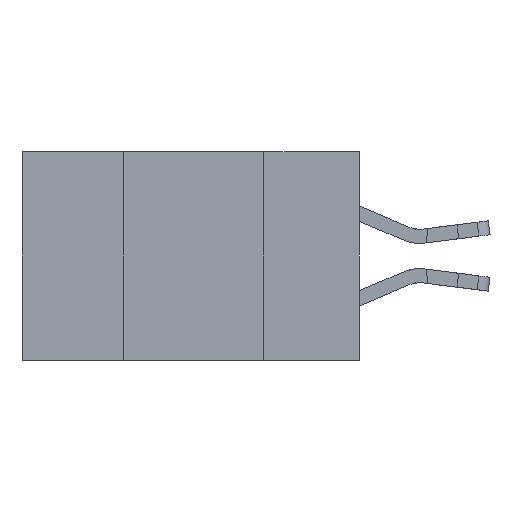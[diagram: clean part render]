
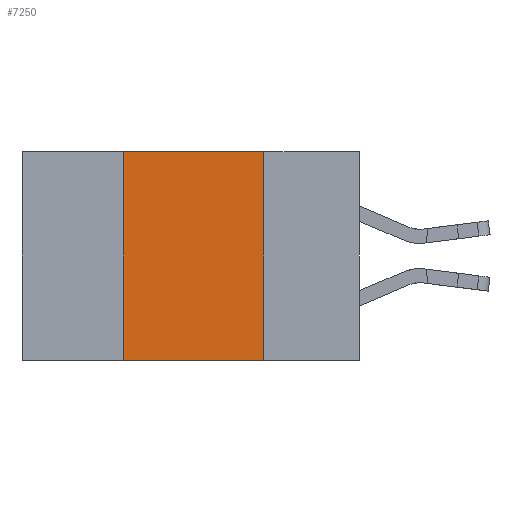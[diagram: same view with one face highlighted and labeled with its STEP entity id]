
A CAD part, left-side view. The second image highlights one B-rep face of the part: STEP entity #7250.
In plain terms, the highlighted planar face has unit normal (-1, 0, 0).
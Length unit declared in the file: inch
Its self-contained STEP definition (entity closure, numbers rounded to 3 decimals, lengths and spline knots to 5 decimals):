
#182 = LINE ( 'NONE', #4715, #15017 ) ;
#208 = VERTEX_POINT ( 'NONE', #18046 ) ;
#451 = EDGE_CURVE ( 'NONE', #5665, #13967, #7849, .T. ) ;
#757 = CARTESIAN_POINT ( 'NONE',  ( 0., 0.6, 0. ) ) ;
#1603 = DIRECTION ( 'NONE',  ( 0., 0., -1. ) ) ;
#2274 = CARTESIAN_POINT ( 'NONE',  ( 0., 0.42, 0. ) ) ;
#3201 = LINE ( 'NONE', #2274, #12126 ) ;
#3503 = VECTOR ( 'NONE', #9624, 39.37008 ) ;
#4179 = ORIENTED_EDGE ( 'NONE', *, *, #10202, .T. ) ;
#4546 = CARTESIAN_POINT ( 'NONE',  ( 0., 0.17, 0. ) ) ;
#4715 = CARTESIAN_POINT ( 'NONE',  ( 0., 0.17, 0. ) ) ;
#5426 = EDGE_LOOP ( 'NONE', ( #12099, #19490, #9662, #4179 ) ) ;
#5665 = VERTEX_POINT ( 'NONE', #16697 ) ;
#6869 = VECTOR ( 'NONE', #13928, 39.37008 ) ;
#7250 = ADVANCED_FACE ( 'NONE', ( #10138 ), #18118, .F. ) ;
#7813 = EDGE_CURVE ( 'NONE', #13967, #208, #182, .T. ) ;
#7849 = LINE ( 'NONE', #12889, #6869 ) ;
#8028 = CARTESIAN_POINT ( 'NONE',  ( 0., 0.6, -0.37 ) ) ;
#8207 = LINE ( 'NONE', #8028, #3503 ) ;
#8714 = DIRECTION ( 'NONE',  ( 1., 0., 0. ) ) ;
#9403 = AXIS2_PLACEMENT_3D ( 'NONE', #757, #8714, #19716 ) ;
#9497 = CARTESIAN_POINT ( 'NONE',  ( 0., 0.42, -0.37 ) ) ;
#9624 = DIRECTION ( 'NONE',  ( 0., -1., 0. ) ) ;
#9662 = ORIENTED_EDGE ( 'NONE', *, *, #13712, .F. ) ;
#10138 = FACE_OUTER_BOUND ( 'NONE', #5426, .T. ) ;
#10202 = EDGE_CURVE ( 'NONE', #17952, #208, #8207, .T. ) ;
#11749 = DIRECTION ( 'NONE',  ( 0., 0., 1. ) ) ;
#12099 = ORIENTED_EDGE ( 'NONE', *, *, #7813, .F. ) ;
#12126 = VECTOR ( 'NONE', #11749, 39.37008 ) ;
#12889 = CARTESIAN_POINT ( 'NONE',  ( 0., 0.6, 0. ) ) ;
#13712 = EDGE_CURVE ( 'NONE', #17952, #5665, #3201, .T. ) ;
#13928 = DIRECTION ( 'NONE',  ( 0., -1., 0. ) ) ;
#13967 = VERTEX_POINT ( 'NONE', #4546 ) ;
#15017 = VECTOR ( 'NONE', #1603, 39.37008 ) ;
#16697 = CARTESIAN_POINT ( 'NONE',  ( 0., 0.42, 0. ) ) ;
#17952 = VERTEX_POINT ( 'NONE', #9497 ) ;
#18046 = CARTESIAN_POINT ( 'NONE',  ( 0., 0.17, -0.37 ) ) ;
#18118 = PLANE ( 'NONE',  #9403 ) ;
#19490 = ORIENTED_EDGE ( 'NONE', *, *, #451, .F. ) ;
#19716 = DIRECTION ( 'NONE',  ( 0., 0., -1. ) ) ;
